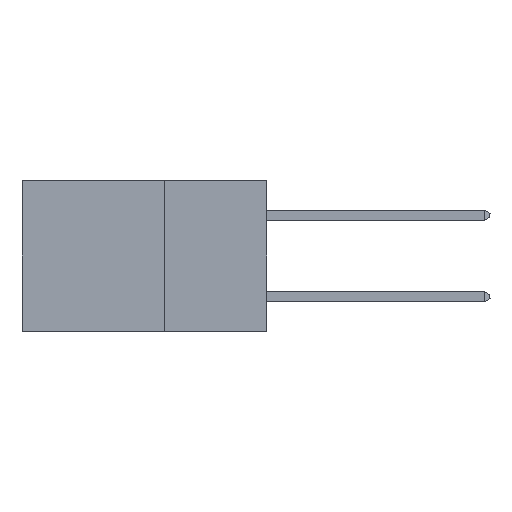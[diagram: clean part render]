
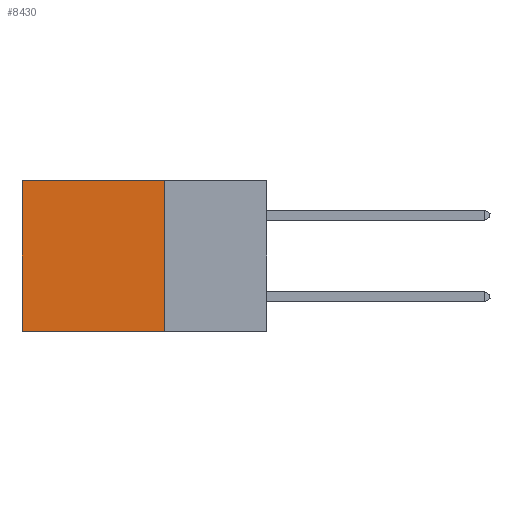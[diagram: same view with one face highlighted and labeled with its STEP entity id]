
A CAD part, left-side view. The second image highlights one B-rep face of the part: STEP entity #8430.
In plain terms, the highlighted planar face has unit normal (-1, 0, 0).
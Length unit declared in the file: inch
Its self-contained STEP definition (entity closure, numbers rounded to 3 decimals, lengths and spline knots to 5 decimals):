
#135 = CARTESIAN_POINT ( 'NONE',  ( 0.2875, 0.25, 0. ) ) ;
#494 = LINE ( 'NONE', #6176, #12018 ) ;
#1554 = CARTESIAN_POINT ( 'NONE',  ( 0.2875, 0.25, -0.37 ) ) ;
#1845 = CARTESIAN_POINT ( 'NONE',  ( 0.2875, 0.25, 0. ) ) ;
#2802 = VECTOR ( 'NONE', #9960, 39.37008 ) ;
#3113 = EDGE_CURVE ( 'NONE', #4563, #6986, #4335, .T. ) ;
#3420 = EDGE_CURVE ( 'NONE', #4563, #16670, #17377, .T. ) ;
#3982 = VECTOR ( 'NONE', #13004, 39.37008 ) ;
#4335 = LINE ( 'NONE', #135, #2802 ) ;
#4563 = VERTEX_POINT ( 'NONE', #12294 ) ;
#4694 = CARTESIAN_POINT ( 'NONE',  ( 0.2875, 0.25, 0. ) ) ;
#4780 = PLANE ( 'NONE',  #13525 ) ;
#4992 = VERTEX_POINT ( 'NONE', #12549 ) ;
#5349 = DIRECTION ( 'NONE',  ( 0., 1., 0. ) ) ;
#5555 = CARTESIAN_POINT ( 'NONE',  ( 0.2875, 0.6, 0. ) ) ;
#6142 = ORIENTED_EDGE ( 'NONE', *, *, #17049, .F. ) ;
#6176 = CARTESIAN_POINT ( 'NONE',  ( 0.2875, 0.6, 0. ) ) ;
#6264 = FACE_OUTER_BOUND ( 'NONE', #11847, .T. ) ;
#6986 = VERTEX_POINT ( 'NONE', #1554 ) ;
#8366 = EDGE_CURVE ( 'NONE', #16670, #4992, #494, .T. ) ;
#8430 = ADVANCED_FACE ( 'NONE', ( #6264 ), #4780, .F. ) ;
#8997 = DIRECTION ( 'NONE',  ( 0., 0., -1. ) ) ;
#9187 = DIRECTION ( 'NONE',  ( 1., 0., 0. ) ) ;
#9960 = DIRECTION ( 'NONE',  ( 0., 0., -1. ) ) ;
#11827 = ORIENTED_EDGE ( 'NONE', *, *, #3113, .F. ) ;
#11847 = EDGE_LOOP ( 'NONE', ( #12006, #6142, #11827, #14983 ) ) ;
#12006 = ORIENTED_EDGE ( 'NONE', *, *, #8366, .T. ) ;
#12018 = VECTOR ( 'NONE', #8997, 39.37008 ) ;
#12294 = CARTESIAN_POINT ( 'NONE',  ( 0.2875, 0.25, 0. ) ) ;
#12549 = CARTESIAN_POINT ( 'NONE',  ( 0.2875, 0.6, -0.37 ) ) ;
#13004 = DIRECTION ( 'NONE',  ( 0., 1., 0. ) ) ;
#13525 = AXIS2_PLACEMENT_3D ( 'NONE', #4694, #9187, #16396 ) ;
#13892 = CARTESIAN_POINT ( 'NONE',  ( 0.2875, 0.25, -0.37 ) ) ;
#14983 = ORIENTED_EDGE ( 'NONE', *, *, #3420, .T. ) ;
#16396 = DIRECTION ( 'NONE',  ( 0., 0., -1. ) ) ;
#16670 = VERTEX_POINT ( 'NONE', #5555 ) ;
#17049 = EDGE_CURVE ( 'NONE', #6986, #4992, #18080, .T. ) ;
#17377 = LINE ( 'NONE', #1845, #3982 ) ;
#18080 = LINE ( 'NONE', #13892, #18447 ) ;
#18447 = VECTOR ( 'NONE', #5349, 39.37008 ) ;
